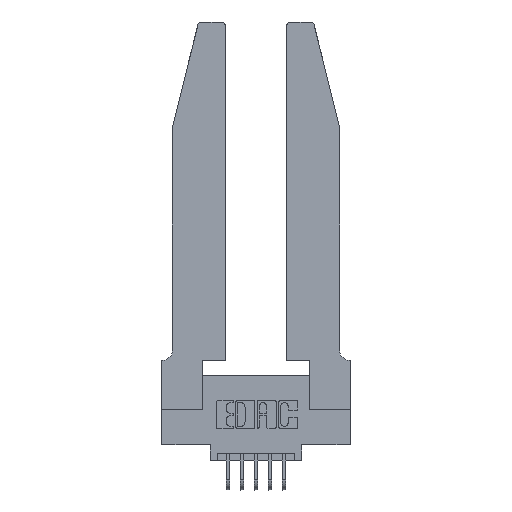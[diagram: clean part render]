
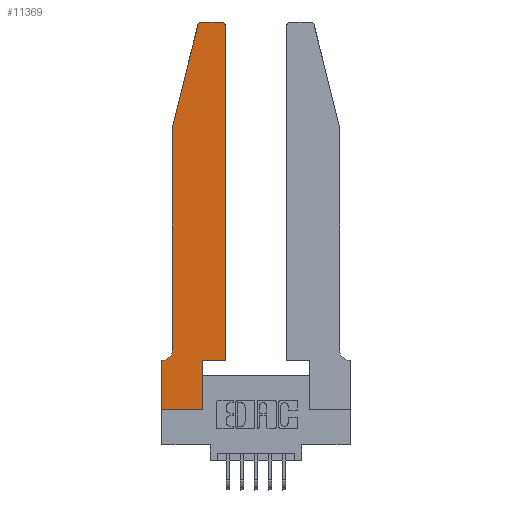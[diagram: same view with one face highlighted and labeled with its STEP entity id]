
A CAD part, top view. The second image highlights one B-rep face of the part: STEP entity #11369.
In plain terms, the highlighted planar face has unit normal (0, 0, 1).
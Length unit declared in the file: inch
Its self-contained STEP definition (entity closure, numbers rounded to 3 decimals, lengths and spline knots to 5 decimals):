
#124 = DIRECTION ( 'NONE',  ( 1., 0., 0. ) ) ;
#160 = EDGE_CURVE ( 'NONE', #4281, #1330, #6816, .T. ) ;
#202 = LINE ( 'NONE', #6495, #8833 ) ;
#376 = CARTESIAN_POINT ( 'NONE',  ( 0., 0.35, 0.37 ) ) ;
#598 = VERTEX_POINT ( 'NONE', #13138 ) ;
#660 = VERTEX_POINT ( 'NONE', #3487 ) ;
#839 = CARTESIAN_POINT ( 'NONE',  ( 0., 0., 0.37 ) ) ;
#862 = CARTESIAN_POINT ( 'NONE',  ( 0.25487, 2.72718, 0.37 ) ) ;
#1044 = LINE ( 'NONE', #10263, #13262 ) ;
#1330 = VERTEX_POINT ( 'NONE', #5074 ) ;
#1611 = ORIENTED_EDGE ( 'NONE', *, *, #13852, .T. ) ;
#1990 = VERTEX_POINT ( 'NONE', #376 ) ;
#2302 = DIRECTION ( 'NONE',  ( 0., -1., 0. ) ) ;
#2385 = EDGE_CURVE ( 'NONE', #12939, #14654, #15384, .T. ) ;
#2408 = CARTESIAN_POINT ( 'NONE',  ( 0.0055, 0.35, 0.37 ) ) ;
#2436 = EDGE_CURVE ( 'NONE', #660, #12939, #5815, .T. ) ;
#2509 = CARTESIAN_POINT ( 'NONE',  ( 0.0055, 0.42, 0.37 ) ) ;
#2532 = CARTESIAN_POINT ( 'NONE',  ( 0., 0., 0.37 ) ) ;
#2538 = VECTOR ( 'NONE', #2302, 39.37008 ) ;
#2567 = VECTOR ( 'NONE', #14273, 39.37008 ) ;
#2724 = ORIENTED_EDGE ( 'NONE', *, *, #8698, .T. ) ;
#2839 = CARTESIAN_POINT ( 'NONE',  ( 0.0755, 2., 0.37 ) ) ;
#2902 = EDGE_CURVE ( 'NONE', #12559, #14640, #15014, .T. ) ;
#2923 = ORIENTED_EDGE ( 'NONE', *, *, #12428, .T. ) ;
#3021 = LINE ( 'NONE', #3148, #15103 ) ;
#3148 = CARTESIAN_POINT ( 'NONE',  ( 0.2865, 0.35, 0.37 ) ) ;
#3160 = CIRCLE ( 'NONE', #8504, 0.03 ) ;
#3221 = DIRECTION ( 'NONE',  ( -0.239, -0.971, 0. ) ) ;
#3484 = EDGE_CURVE ( 'NONE', #1990, #4281, #5788, .T. ) ;
#3487 = CARTESIAN_POINT ( 'NONE',  ( 0.4205, 2.75, 0.37 ) ) ;
#3575 = VECTOR ( 'NONE', #7651, 39.37008 ) ;
#3770 = DIRECTION ( 'NONE',  ( -1., 0., 0. ) ) ;
#3859 = AXIS2_PLACEMENT_3D ( 'NONE', #13149, #8669, #124 ) ;
#3885 = CIRCLE ( 'NONE', #14290, 0.07 ) ;
#4281 = VERTEX_POINT ( 'NONE', #8924 ) ;
#4830 = ORIENTED_EDGE ( 'NONE', *, *, #2902, .T. ) ;
#5074 = CARTESIAN_POINT ( 'NONE',  ( 0.2865, 0., 0.37 ) ) ;
#5144 = FACE_OUTER_BOUND ( 'NONE', #13200, .T. ) ;
#5201 = ORIENTED_EDGE ( 'NONE', *, *, #9735, .T. ) ;
#5228 = VECTOR ( 'NONE', #9227, 39.37008 ) ;
#5370 = AXIS2_PLACEMENT_3D ( 'NONE', #14003, #11959, #10499 ) ;
#5788 = LINE ( 'NONE', #2532, #2538 ) ;
#5815 = LINE ( 'NONE', #14862, #2567 ) ;
#5885 = ORIENTED_EDGE ( 'NONE', *, *, #14367, .T. ) ;
#6165 = EDGE_CURVE ( 'NONE', #1330, #14513, #3021, .T. ) ;
#6277 = VERTEX_POINT ( 'NONE', #2408 ) ;
#6318 = DIRECTION ( 'NONE',  ( 0., 0., 1. ) ) ;
#6495 = CARTESIAN_POINT ( 'NONE',  ( 0.4505, 0.35, 0.37 ) ) ;
#6816 = LINE ( 'NONE', #839, #3575 ) ;
#6843 = DIRECTION ( 'NONE',  ( 0., 1., 0. ) ) ;
#7166 = ORIENTED_EDGE ( 'NONE', *, *, #7818, .T. ) ;
#7651 = DIRECTION ( 'NONE',  ( 1., 0., 0. ) ) ;
#7686 = DIRECTION ( 'NONE',  ( 0., 1., 0. ) ) ;
#7818 = EDGE_CURVE ( 'NONE', #14513, #598, #14035, .T. ) ;
#8136 = LINE ( 'NONE', #9998, #13815 ) ;
#8504 = AXIS2_PLACEMENT_3D ( 'NONE', #13164, #6318, #14329 ) ;
#8669 = DIRECTION ( 'NONE',  ( 0., 0., 1. ) ) ;
#8698 = EDGE_CURVE ( 'NONE', #14640, #6277, #3885, .T. ) ;
#8833 = VECTOR ( 'NONE', #7686, 39.37008 ) ;
#8878 = VECTOR ( 'NONE', #14081, 39.37008 ) ;
#8924 = CARTESIAN_POINT ( 'NONE',  ( 0., 0., 0.37 ) ) ;
#9227 = DIRECTION ( 'NONE',  ( 1., 0., 0. ) ) ;
#9735 = EDGE_CURVE ( 'NONE', #14654, #12559, #1044, .T. ) ;
#9998 = CARTESIAN_POINT ( 'NONE',  ( 0.0755, 0.35, 0.37 ) ) ;
#10032 = CARTESIAN_POINT ( 'NONE',  ( 0.4505, 2.72, 0.37 ) ) ;
#10263 = CARTESIAN_POINT ( 'NONE',  ( 0.0755, 2., 0.37 ) ) ;
#10292 = ORIENTED_EDGE ( 'NONE', *, *, #3484, .T. ) ;
#10499 = DIRECTION ( 'NONE',  ( 1., 0., 0. ) ) ;
#10759 = DIRECTION ( 'NONE',  ( 0., 0., -1. ) ) ;
#11179 = DIRECTION ( 'NONE',  ( -1., 0., 0. ) ) ;
#11369 = ADVANCED_FACE ( 'NONE', ( #5144 ), #13242, .T. ) ;
#11782 = ORIENTED_EDGE ( 'NONE', *, *, #160, .T. ) ;
#11959 = DIRECTION ( 'NONE',  ( 0., 0., 1. ) ) ;
#12428 = EDGE_CURVE ( 'NONE', #15068, #660, #3160, .T. ) ;
#12559 = VERTEX_POINT ( 'NONE', #2839 ) ;
#12663 = CARTESIAN_POINT ( 'NONE',  ( 0.4505, 0.35, 0.37 ) ) ;
#12692 = CARTESIAN_POINT ( 'NONE',  ( 0.0755, 0.42, 0.37 ) ) ;
#12939 = VERTEX_POINT ( 'NONE', #14006 ) ;
#13083 = ORIENTED_EDGE ( 'NONE', *, *, #2436, .T. ) ;
#13138 = CARTESIAN_POINT ( 'NONE',  ( 0.4505, 0.35, 0.37 ) ) ;
#13149 = CARTESIAN_POINT ( 'NONE',  ( 0., 0.35, 0.37 ) ) ;
#13164 = CARTESIAN_POINT ( 'NONE',  ( 0.4205, 2.72, 0.37 ) ) ;
#13200 = EDGE_LOOP ( 'NONE', ( #13083, #14103, #5201, #4830, #2724, #5885, #10292, #11782, #14198, #7166, #1611, #2923 ) ) ;
#13242 = PLANE ( 'NONE',  #3859 ) ;
#13262 = VECTOR ( 'NONE', #3221, 39.37008 ) ;
#13795 = CARTESIAN_POINT ( 'NONE',  ( 0.0755, 2., 0.37 ) ) ;
#13815 = VECTOR ( 'NONE', #11179, 39.37008 ) ;
#13852 = EDGE_CURVE ( 'NONE', #598, #15068, #202, .T. ) ;
#14003 = CARTESIAN_POINT ( 'NONE',  ( 0.284, 2.72, 0.37 ) ) ;
#14006 = CARTESIAN_POINT ( 'NONE',  ( 0.284, 2.75, 0.37 ) ) ;
#14035 = LINE ( 'NONE', #12663, #5228 ) ;
#14081 = DIRECTION ( 'NONE',  ( 0., -1., 0. ) ) ;
#14103 = ORIENTED_EDGE ( 'NONE', *, *, #2385, .T. ) ;
#14198 = ORIENTED_EDGE ( 'NONE', *, *, #6165, .T. ) ;
#14273 = DIRECTION ( 'NONE',  ( -1., 0., 0. ) ) ;
#14290 = AXIS2_PLACEMENT_3D ( 'NONE', #2509, #10759, #3770 ) ;
#14329 = DIRECTION ( 'NONE',  ( 1., 0., 0. ) ) ;
#14367 = EDGE_CURVE ( 'NONE', #6277, #1990, #8136, .T. ) ;
#14513 = VERTEX_POINT ( 'NONE', #14797 ) ;
#14640 = VERTEX_POINT ( 'NONE', #12692 ) ;
#14654 = VERTEX_POINT ( 'NONE', #862 ) ;
#14797 = CARTESIAN_POINT ( 'NONE',  ( 0.2865, 0.35, 0.37 ) ) ;
#14862 = CARTESIAN_POINT ( 'NONE',  ( 0.2605, 2.75, 0.37 ) ) ;
#15014 = LINE ( 'NONE', #13795, #8878 ) ;
#15068 = VERTEX_POINT ( 'NONE', #10032 ) ;
#15103 = VECTOR ( 'NONE', #6843, 39.37008 ) ;
#15384 = CIRCLE ( 'NONE', #5370, 0.03 ) ;
